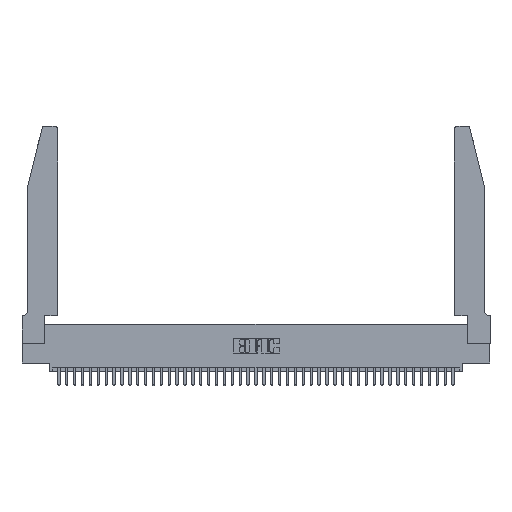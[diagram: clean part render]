
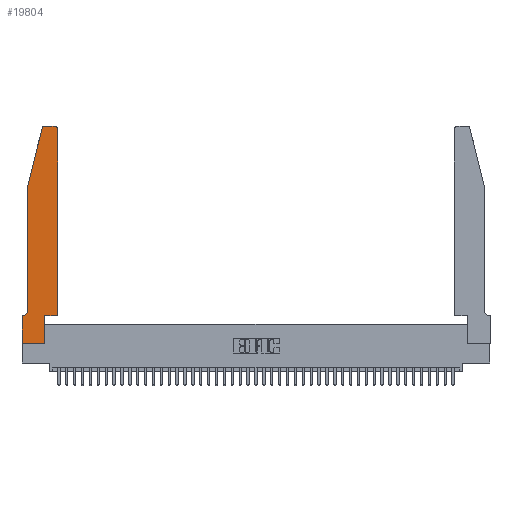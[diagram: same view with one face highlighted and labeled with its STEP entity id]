
A CAD part, top view. The second image highlights one B-rep face of the part: STEP entity #19804.
In plain terms, the highlighted planar face has unit normal (0, 0, 1).
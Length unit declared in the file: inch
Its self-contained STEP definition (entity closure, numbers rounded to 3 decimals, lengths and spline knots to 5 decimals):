
#8 = VECTOR ( 'NONE', #23888, 39.37008 ) ;
#694 = LINE ( 'NONE', #41779, #35612 ) ;
#1168 = VERTEX_POINT ( 'NONE', #17550 ) ;
#1499 = DIRECTION ( 'NONE',  ( 0., 1., 0. ) ) ;
#2796 = FACE_OUTER_BOUND ( 'NONE', #11294, .T. ) ;
#2893 = DIRECTION ( 'NONE',  ( 1., 0., 0. ) ) ;
#3422 = CARTESIAN_POINT ( 'NONE',  ( 0.2865, 0.35, 0.37 ) ) ;
#4192 = VERTEX_POINT ( 'NONE', #32623 ) ;
#5110 = VERTEX_POINT ( 'NONE', #27142 ) ;
#5394 = EDGE_CURVE ( 'NONE', #15201, #25266, #5662, .T. ) ;
#5662 = LINE ( 'NONE', #33568, #31583 ) ;
#6156 = EDGE_CURVE ( 'NONE', #25266, #13164, #33143, .T. ) ;
#6346 = LINE ( 'NONE', #35357, #32298 ) ;
#7263 = ORIENTED_EDGE ( 'NONE', *, *, #38715, .T. ) ;
#7306 = CARTESIAN_POINT ( 'NONE',  ( 0.4205, 2.75, 0.37 ) ) ;
#7968 = VERTEX_POINT ( 'NONE', #35675 ) ;
#8277 = DIRECTION ( 'NONE',  ( 1., 0., 0. ) ) ;
#9184 = AXIS2_PLACEMENT_3D ( 'NONE', #24882, #18249, #35084 ) ;
#9767 = CARTESIAN_POINT ( 'NONE',  ( 0.2865, 0., 0.37 ) ) ;
#9903 = ORIENTED_EDGE ( 'NONE', *, *, #19028, .T. ) ;
#11294 = EDGE_LOOP ( 'NONE', ( #26425, #43334, #9903, #36890, #35679, #7263, #42389, #39430, #11322, #36915, #27421, #41324 ) ) ;
#11322 = ORIENTED_EDGE ( 'NONE', *, *, #11584, .T. ) ;
#11517 = PLANE ( 'NONE',  #18202 ) ;
#11584 = EDGE_CURVE ( 'NONE', #37340, #5110, #42110, .T. ) ;
#12274 = DIRECTION ( 'NONE',  ( 0., 0., -1. ) ) ;
#12388 = CIRCLE ( 'NONE', #9184, 0.03 ) ;
#12750 = VERTEX_POINT ( 'NONE', #19211 ) ;
#13122 = EDGE_CURVE ( 'NONE', #7968, #4192, #694, .T. ) ;
#13164 = VERTEX_POINT ( 'NONE', #18285 ) ;
#13473 = LINE ( 'NONE', #18299, #33063 ) ;
#15201 = VERTEX_POINT ( 'NONE', #7306 ) ;
#17550 = CARTESIAN_POINT ( 'NONE',  ( 0.4505, 0.35, 0.37 ) ) ;
#18076 = CARTESIAN_POINT ( 'NONE',  ( 0.0755, 2., 0.37 ) ) ;
#18202 = AXIS2_PLACEMENT_3D ( 'NONE', #21322, #21772, #24729 ) ;
#18249 = DIRECTION ( 'NONE',  ( 0., 0., 1. ) ) ;
#18285 = CARTESIAN_POINT ( 'NONE',  ( 0.25487, 2.72718, 0.37 ) ) ;
#18299 = CARTESIAN_POINT ( 'NONE',  ( 0., 0., 0.37 ) ) ;
#18317 = VECTOR ( 'NONE', #19840, 39.37008 ) ;
#18550 = LINE ( 'NONE', #30496, #8 ) ;
#19028 = EDGE_CURVE ( 'NONE', #13164, #39132, #43586, .T. ) ;
#19211 = CARTESIAN_POINT ( 'NONE',  ( 0.0055, 0.35, 0.37 ) ) ;
#19274 = CARTESIAN_POINT ( 'NONE',  ( 0.0055, 0.42, 0.37 ) ) ;
#19804 = ADVANCED_FACE ( 'NONE', ( #2796 ), #11517, .T. ) ;
#19840 = DIRECTION ( 'NONE',  ( 0., 1., 0. ) ) ;
#20172 = VECTOR ( 'NONE', #2893, 39.37008 ) ;
#21322 = CARTESIAN_POINT ( 'NONE',  ( 0., 0.35, 0.37 ) ) ;
#21772 = DIRECTION ( 'NONE',  ( 0., 0., 1. ) ) ;
#21835 = EDGE_CURVE ( 'NONE', #39132, #22883, #39342, .T. ) ;
#22883 = VERTEX_POINT ( 'NONE', #43729 ) ;
#23888 = DIRECTION ( 'NONE',  ( -1., 0., 0. ) ) ;
#24525 = EDGE_CURVE ( 'NONE', #1168, #27481, #6346, .T. ) ;
#24729 = DIRECTION ( 'NONE',  ( 1., 0., 0. ) ) ;
#24882 = CARTESIAN_POINT ( 'NONE',  ( 0.4205, 2.72, 0.37 ) ) ;
#24997 = DIRECTION ( 'NONE',  ( 0., -1., 0. ) ) ;
#25266 = VERTEX_POINT ( 'NONE', #31129 ) ;
#25909 = CARTESIAN_POINT ( 'NONE',  ( 0.0755, 2., 0.37 ) ) ;
#26425 = ORIENTED_EDGE ( 'NONE', *, *, #5394, .T. ) ;
#26517 = DIRECTION ( 'NONE',  ( -0.239, -0.971, 0. ) ) ;
#27132 = AXIS2_PLACEMENT_3D ( 'NONE', #19274, #12274, #29122 ) ;
#27142 = CARTESIAN_POINT ( 'NONE',  ( 0.2865, 0.35, 0.37 ) ) ;
#27421 = ORIENTED_EDGE ( 'NONE', *, *, #24525, .T. ) ;
#27481 = VERTEX_POINT ( 'NONE', #35685 ) ;
#28119 = EDGE_CURVE ( 'NONE', #22883, #12750, #32017, .T. ) ;
#28527 = CARTESIAN_POINT ( 'NONE',  ( 0.284, 2.72, 0.37 ) ) ;
#29122 = DIRECTION ( 'NONE',  ( -1., 0., 0. ) ) ;
#30033 = CARTESIAN_POINT ( 'NONE',  ( 0.0755, 2., 0.37 ) ) ;
#30496 = CARTESIAN_POINT ( 'NONE',  ( 0.0755, 0.35, 0.37 ) ) ;
#30946 = EDGE_CURVE ( 'NONE', #5110, #1168, #33398, .T. ) ;
#31129 = CARTESIAN_POINT ( 'NONE',  ( 0.284, 2.75, 0.37 ) ) ;
#31583 = VECTOR ( 'NONE', #33004, 39.37008 ) ;
#32017 = CIRCLE ( 'NONE', #27132, 0.07 ) ;
#32298 = VECTOR ( 'NONE', #1499, 39.37008 ) ;
#32623 = CARTESIAN_POINT ( 'NONE',  ( 0., 0., 0.37 ) ) ;
#33004 = DIRECTION ( 'NONE',  ( -1., 0., 0. ) ) ;
#33063 = VECTOR ( 'NONE', #34685, 39.37008 ) ;
#33143 = CIRCLE ( 'NONE', #35752, 0.03 ) ;
#33398 = LINE ( 'NONE', #43409, #20172 ) ;
#33568 = CARTESIAN_POINT ( 'NONE',  ( 0.2605, 2.75, 0.37 ) ) ;
#34685 = DIRECTION ( 'NONE',  ( 1., 0., 0. ) ) ;
#34813 = DIRECTION ( 'NONE',  ( 0., -1., 0. ) ) ;
#35084 = DIRECTION ( 'NONE',  ( 1., 0., 0. ) ) ;
#35357 = CARTESIAN_POINT ( 'NONE',  ( 0.4505, 0.35, 0.37 ) ) ;
#35368 = DIRECTION ( 'NONE',  ( 0., 0., 1. ) ) ;
#35612 = VECTOR ( 'NONE', #34813, 39.37008 ) ;
#35650 = VECTOR ( 'NONE', #24997, 39.37008 ) ;
#35675 = CARTESIAN_POINT ( 'NONE',  ( 0., 0.35, 0.37 ) ) ;
#35679 = ORIENTED_EDGE ( 'NONE', *, *, #28119, .T. ) ;
#35685 = CARTESIAN_POINT ( 'NONE',  ( 0.4505, 2.72, 0.37 ) ) ;
#35752 = AXIS2_PLACEMENT_3D ( 'NONE', #28527, #35368, #8277 ) ;
#35908 = EDGE_CURVE ( 'NONE', #4192, #37340, #13473, .T. ) ;
#36483 = EDGE_CURVE ( 'NONE', #27481, #15201, #12388, .T. ) ;
#36890 = ORIENTED_EDGE ( 'NONE', *, *, #21835, .T. ) ;
#36915 = ORIENTED_EDGE ( 'NONE', *, *, #30946, .T. ) ;
#37340 = VERTEX_POINT ( 'NONE', #9767 ) ;
#38261 = VECTOR ( 'NONE', #26517, 39.37008 ) ;
#38715 = EDGE_CURVE ( 'NONE', #12750, #7968, #18550, .T. ) ;
#39132 = VERTEX_POINT ( 'NONE', #25909 ) ;
#39342 = LINE ( 'NONE', #18076, #35650 ) ;
#39430 = ORIENTED_EDGE ( 'NONE', *, *, #35908, .T. ) ;
#41324 = ORIENTED_EDGE ( 'NONE', *, *, #36483, .T. ) ;
#41779 = CARTESIAN_POINT ( 'NONE',  ( 0., 0., 0.37 ) ) ;
#42110 = LINE ( 'NONE', #3422, #18317 ) ;
#42389 = ORIENTED_EDGE ( 'NONE', *, *, #13122, .T. ) ;
#43334 = ORIENTED_EDGE ( 'NONE', *, *, #6156, .T. ) ;
#43409 = CARTESIAN_POINT ( 'NONE',  ( 0.4505, 0.35, 0.37 ) ) ;
#43586 = LINE ( 'NONE', #30033, #38261 ) ;
#43729 = CARTESIAN_POINT ( 'NONE',  ( 0.0755, 0.42, 0.37 ) ) ;
